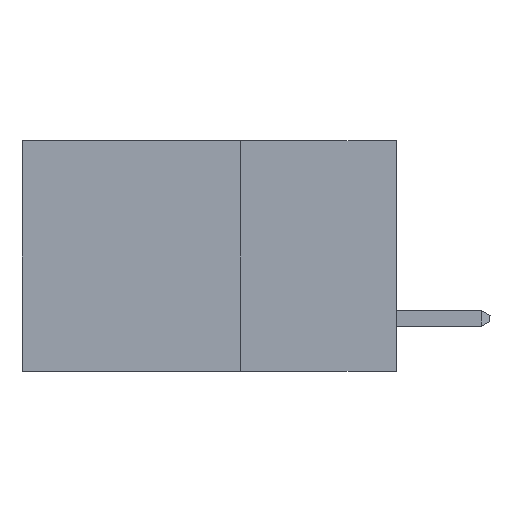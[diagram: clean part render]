
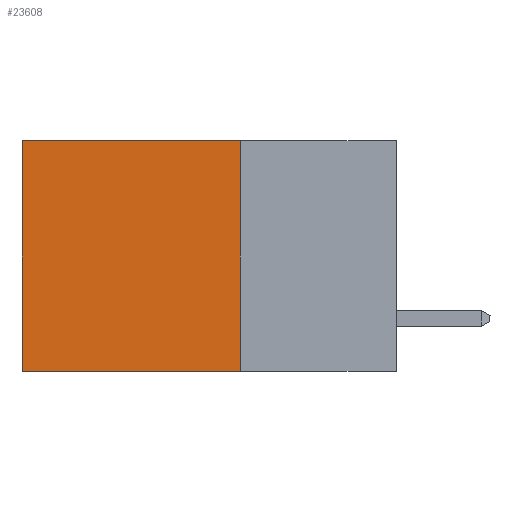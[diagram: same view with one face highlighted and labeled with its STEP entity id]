
A CAD part, left-side view. The second image highlights one B-rep face of the part: STEP entity #23608.
In plain terms, the highlighted planar face has unit normal (-1, 0, 0).
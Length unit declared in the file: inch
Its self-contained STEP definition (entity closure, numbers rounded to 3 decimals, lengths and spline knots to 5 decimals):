
#811 = PLANE ( 'NONE',  #15551 ) ;
#2432 = LINE ( 'NONE', #6511, #6816 ) ;
#2591 = EDGE_CURVE ( 'NONE', #22256, #8445, #10593, .T. ) ;
#2754 = CARTESIAN_POINT ( 'NONE',  ( 0.2615, 0.25, -0.37 ) ) ;
#4456 = EDGE_CURVE ( 'NONE', #22256, #4925, #9679, .T. ) ;
#4702 = VECTOR ( 'NONE', #8464, 39.37008 ) ;
#4925 = VERTEX_POINT ( 'NONE', #21490 ) ;
#5167 = CARTESIAN_POINT ( 'NONE',  ( 0.2615, 0.6, -0.37 ) ) ;
#5450 = ORIENTED_EDGE ( 'NONE', *, *, #2591, .F. ) ;
#5734 = CARTESIAN_POINT ( 'NONE',  ( 0.2615, 0.25, 0. ) ) ;
#6148 = ORIENTED_EDGE ( 'NONE', *, *, #9352, .T. ) ;
#6424 = DIRECTION ( 'NONE',  ( 0., 0., -1. ) ) ;
#6511 = CARTESIAN_POINT ( 'NONE',  ( 0.2615, 0.6, -0.37 ) ) ;
#6816 = VECTOR ( 'NONE', #8770, 39.37008 ) ;
#7157 = EDGE_LOOP ( 'NONE', ( #6148, #24643, #5450, #9869 ) ) ;
#8445 = VERTEX_POINT ( 'NONE', #15647 ) ;
#8464 = DIRECTION ( 'NONE',  ( 0., 1., 0. ) ) ;
#8770 = DIRECTION ( 'NONE',  ( 0., 0., -1. ) ) ;
#8820 = DIRECTION ( 'NONE',  ( 1., 0., 0. ) ) ;
#9352 = EDGE_CURVE ( 'NONE', #4925, #21775, #2432, .T. ) ;
#9679 = LINE ( 'NONE', #5734, #19111 ) ;
#9869 = ORIENTED_EDGE ( 'NONE', *, *, #4456, .T. ) ;
#10593 = LINE ( 'NONE', #2754, #17452 ) ;
#10732 = DIRECTION ( 'NONE',  ( 0., 0., -1. ) ) ;
#10923 = EDGE_CURVE ( 'NONE', #8445, #21775, #20381, .T. ) ;
#12775 = CARTESIAN_POINT ( 'NONE',  ( 0.2615, 0.25, -0.37 ) ) ;
#15551 = AXIS2_PLACEMENT_3D ( 'NONE', #24773, #8820, #6424 ) ;
#15647 = CARTESIAN_POINT ( 'NONE',  ( 0.2615, 0.25, -0.37 ) ) ;
#16449 = CARTESIAN_POINT ( 'NONE',  ( 0.2615, 0.25, 0. ) ) ;
#17452 = VECTOR ( 'NONE', #10732, 39.37008 ) ;
#18656 = FACE_OUTER_BOUND ( 'NONE', #7157, .T. ) ;
#19111 = VECTOR ( 'NONE', #19148, 39.37008 ) ;
#19148 = DIRECTION ( 'NONE',  ( 0., 1., 0. ) ) ;
#20381 = LINE ( 'NONE', #12775, #4702 ) ;
#21490 = CARTESIAN_POINT ( 'NONE',  ( 0.2615, 0.6, 0. ) ) ;
#21775 = VERTEX_POINT ( 'NONE', #5167 ) ;
#22256 = VERTEX_POINT ( 'NONE', #16449 ) ;
#23608 = ADVANCED_FACE ( 'NONE', ( #18656 ), #811, .F. ) ;
#24643 = ORIENTED_EDGE ( 'NONE', *, *, #10923, .F. ) ;
#24773 = CARTESIAN_POINT ( 'NONE',  ( 0.2615, 0.25, -0.37 ) ) ;
